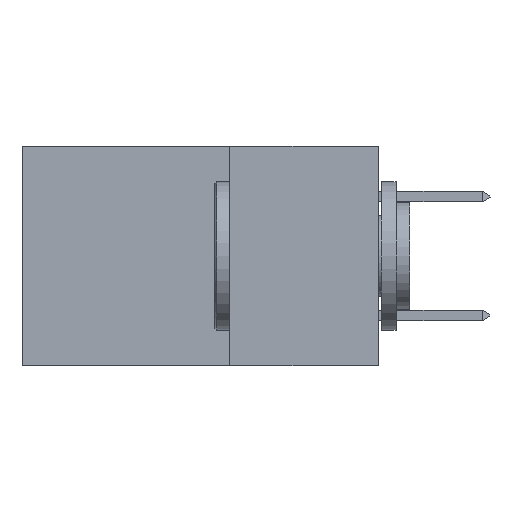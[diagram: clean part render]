
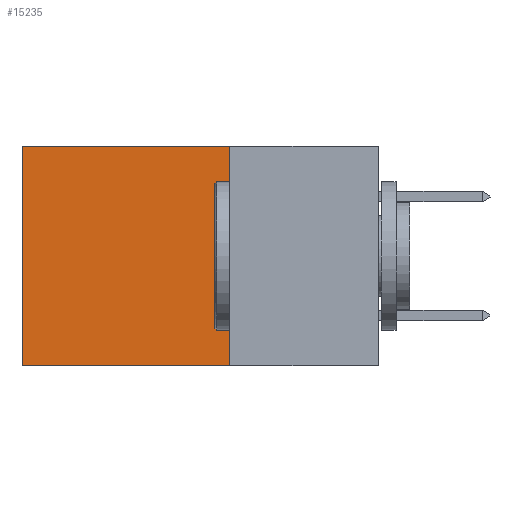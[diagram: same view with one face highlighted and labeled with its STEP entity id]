
A CAD part, left-side view. The second image highlights one B-rep face of the part: STEP entity #15235.
In plain terms, the highlighted planar face has unit normal (-1, 0, 0).
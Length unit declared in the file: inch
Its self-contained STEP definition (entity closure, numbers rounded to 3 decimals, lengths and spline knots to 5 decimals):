
#55 = LINE ( 'NONE', #23363, #27934 ) ;
#80 = DIRECTION ( 'NONE',  ( 1., 0., 0. ) ) ;
#487 = VECTOR ( 'NONE', #7882, 39.37008 ) ;
#1388 = CARTESIAN_POINT ( 'NONE',  ( 0.298, 0.25, 0. ) ) ;
#2302 = EDGE_CURVE ( 'NONE', #25317, #7475, #8098, .T. ) ;
#3617 = CARTESIAN_POINT ( 'NONE',  ( 0.298, 0.6, 0. ) ) ;
#4894 = DIRECTION ( 'NONE',  ( 0., 1., 0. ) ) ;
#6620 = CARTESIAN_POINT ( 'NONE',  ( 0.298, 0.25, -0.37 ) ) ;
#6829 = EDGE_CURVE ( 'NONE', #8788, #28363, #55, .T. ) ;
#7475 = VERTEX_POINT ( 'NONE', #25245 ) ;
#7882 = DIRECTION ( 'NONE',  ( 0., 0., -1. ) ) ;
#8098 = LINE ( 'NONE', #6620, #27015 ) ;
#8674 = CARTESIAN_POINT ( 'NONE',  ( 0.298, 0.6, 0. ) ) ;
#8788 = VERTEX_POINT ( 'NONE', #17146 ) ;
#8878 = DIRECTION ( 'NONE',  ( 0., 0., -1. ) ) ;
#9249 = VECTOR ( 'NONE', #8878, 39.37008 ) ;
#10049 = EDGE_LOOP ( 'NONE', ( #25306, #10084, #14005, #24426 ) ) ;
#10084 = ORIENTED_EDGE ( 'NONE', *, *, #2302, .F. ) ;
#11075 = DIRECTION ( 'NONE',  ( 0., 1., 0. ) ) ;
#11794 = DIRECTION ( 'NONE',  ( 0., 0., -1. ) ) ;
#12550 = CARTESIAN_POINT ( 'NONE',  ( 0.298, 0.25, -0.37 ) ) ;
#12714 = EDGE_CURVE ( 'NONE', #28363, #7475, #13519, .T. ) ;
#12808 = AXIS2_PLACEMENT_3D ( 'NONE', #1388, #80, #11794 ) ;
#13519 = LINE ( 'NONE', #8674, #9249 ) ;
#14005 = ORIENTED_EDGE ( 'NONE', *, *, #19442, .F. ) ;
#15235 = ADVANCED_FACE ( 'NONE', ( #17198 ), #31453, .F. ) ;
#17146 = CARTESIAN_POINT ( 'NONE',  ( 0.298, 0.25, 0. ) ) ;
#17198 = FACE_OUTER_BOUND ( 'NONE', #10049, .T. ) ;
#19442 = EDGE_CURVE ( 'NONE', #8788, #25317, #31830, .T. ) ;
#23363 = CARTESIAN_POINT ( 'NONE',  ( 0.298, 0.25, 0. ) ) ;
#24426 = ORIENTED_EDGE ( 'NONE', *, *, #6829, .T. ) ;
#25245 = CARTESIAN_POINT ( 'NONE',  ( 0.298, 0.6, -0.37 ) ) ;
#25306 = ORIENTED_EDGE ( 'NONE', *, *, #12714, .T. ) ;
#25317 = VERTEX_POINT ( 'NONE', #12550 ) ;
#27015 = VECTOR ( 'NONE', #4894, 39.37008 ) ;
#27426 = CARTESIAN_POINT ( 'NONE',  ( 0.298, 0.25, 0. ) ) ;
#27934 = VECTOR ( 'NONE', #11075, 39.37008 ) ;
#28363 = VERTEX_POINT ( 'NONE', #3617 ) ;
#31453 = PLANE ( 'NONE',  #12808 ) ;
#31830 = LINE ( 'NONE', #27426, #487 ) ;
